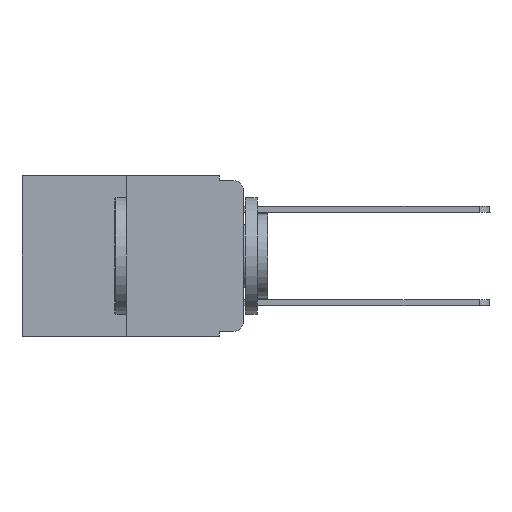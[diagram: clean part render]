
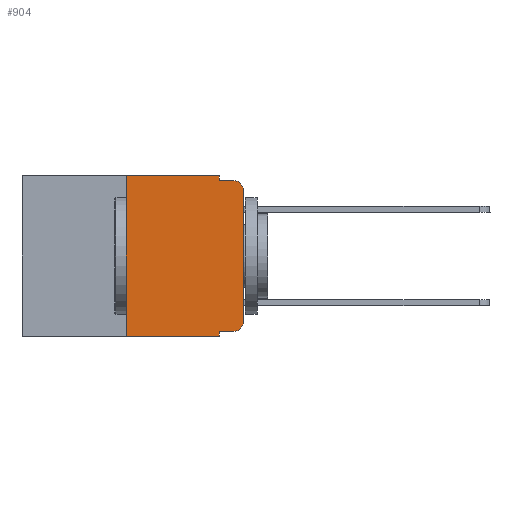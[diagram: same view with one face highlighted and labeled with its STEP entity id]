
A CAD part, left-side view. The second image highlights one B-rep face of the part: STEP entity #904.
In plain terms, the highlighted planar face has unit normal (-1, 0, 0).
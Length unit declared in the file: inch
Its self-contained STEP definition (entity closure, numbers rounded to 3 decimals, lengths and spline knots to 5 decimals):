
#121 = EDGE_CURVE ( 'NONE', #17279, #10276, #17104, .T. ) ;
#374 = CARTESIAN_POINT ( 'NONE',  ( 0., 0.051, -0.333 ) ) ;
#904 = ADVANCED_FACE ( 'NONE', ( #21860 ), #13924, .F. ) ;
#1148 = CARTESIAN_POINT ( 'NONE',  ( 0., 0.473, 0. ) ) ;
#1554 = CIRCLE ( 'NONE', #14560, 0.02 ) ;
#1860 = DIRECTION ( 'NONE',  ( 0., 0., -1. ) ) ;
#1947 = EDGE_CURVE ( 'NONE', #19903, #21428, #14123, .T. ) ;
#2002 = AXIS2_PLACEMENT_3D ( 'NONE', #1148, #24027, #9707 ) ;
#2800 = VECTOR ( 'NONE', #18866, 39.37008 ) ;
#2885 = EDGE_LOOP ( 'NONE', ( #4805, #8491, #22741, #19650, #20838, #8786, #24686, #14273, #6518, #10645 ) ) ;
#3373 = DIRECTION ( 'NONE',  ( -1., 0., 0. ) ) ;
#3546 = VECTOR ( 'NONE', #3890, 39.37008 ) ;
#3624 = CARTESIAN_POINT ( 'NONE',  ( 0., 0., 0. ) ) ;
#3808 = DIRECTION ( 'NONE',  ( 0., -1., 0. ) ) ;
#3831 = CARTESIAN_POINT ( 'NONE',  ( 0., 0.051, 0. ) ) ;
#3858 = VECTOR ( 'NONE', #16967, 39.37008 ) ;
#3890 = DIRECTION ( 'NONE',  ( 0., 0., 1. ) ) ;
#4146 = CARTESIAN_POINT ( 'NONE',  ( 0., 0.051, 0. ) ) ;
#4435 = CARTESIAN_POINT ( 'NONE',  ( 0., 0.25, 0. ) ) ;
#4805 = ORIENTED_EDGE ( 'NONE', *, *, #13808, .T. ) ;
#4909 = EDGE_CURVE ( 'NONE', #5352, #11208, #15163, .T. ) ;
#5352 = VERTEX_POINT ( 'NONE', #6668 ) ;
#5969 = EDGE_CURVE ( 'NONE', #20537, #21428, #16666, .T. ) ;
#6219 = EDGE_CURVE ( 'NONE', #18293, #5352, #23092, .T. ) ;
#6518 = ORIENTED_EDGE ( 'NONE', *, *, #121, .T. ) ;
#6668 = CARTESIAN_POINT ( 'NONE',  ( 0., 0.25, 0. ) ) ;
#7770 = DIRECTION ( 'NONE',  ( 0., 0., -1. ) ) ;
#7827 = LINE ( 'NONE', #3624, #3546 ) ;
#7944 = VECTOR ( 'NONE', #20354, 39.37008 ) ;
#7961 = DIRECTION ( 'NONE',  ( 0., 0., -1. ) ) ;
#8485 = LINE ( 'NONE', #4146, #21129 ) ;
#8491 = ORIENTED_EDGE ( 'NONE', *, *, #5969, .T. ) ;
#8589 = CARTESIAN_POINT ( 'NONE',  ( 0., 0., -0.313 ) ) ;
#8786 = ORIENTED_EDGE ( 'NONE', *, *, #6219, .F. ) ;
#9242 = CARTESIAN_POINT ( 'NONE',  ( 0., 0.051, -0.01 ) ) ;
#9655 = CARTESIAN_POINT ( 'NONE',  ( 0., 0.02, -0.333 ) ) ;
#9665 = LINE ( 'NONE', #3831, #10511 ) ;
#9701 = CARTESIAN_POINT ( 'NONE',  ( 0., 0.473, -0.343 ) ) ;
#9707 = DIRECTION ( 'NONE',  ( 0., 0., -1. ) ) ;
#10141 = VERTEX_POINT ( 'NONE', #8589 ) ;
#10276 = VERTEX_POINT ( 'NONE', #9655 ) ;
#10511 = VECTOR ( 'NONE', #7770, 39.37008 ) ;
#10645 = ORIENTED_EDGE ( 'NONE', *, *, #21133, .T. ) ;
#11208 = VERTEX_POINT ( 'NONE', #21876 ) ;
#11214 = CARTESIAN_POINT ( 'NONE',  ( 0., 0.473, 0. ) ) ;
#13629 = AXIS2_PLACEMENT_3D ( 'NONE', #22030, #3373, #1860 ) ;
#13663 = VECTOR ( 'NONE', #19404, 39.37008 ) ;
#13808 = EDGE_CURVE ( 'NONE', #10141, #20537, #7827, .T. ) ;
#13924 = PLANE ( 'NONE',  #2002 ) ;
#14011 = CARTESIAN_POINT ( 'NONE',  ( 0., 0.02, -0.01 ) ) ;
#14118 = VECTOR ( 'NONE', #3808, 39.37008 ) ;
#14123 = LINE ( 'NONE', #24493, #14118 ) ;
#14273 = ORIENTED_EDGE ( 'NONE', *, *, #16043, .F. ) ;
#14560 = AXIS2_PLACEMENT_3D ( 'NONE', #16646, #26639, #7961 ) ;
#15078 = CARTESIAN_POINT ( 'NONE',  ( 0., 0.051, -0.343 ) ) ;
#15163 = LINE ( 'NONE', #11214, #13663 ) ;
#16043 = EDGE_CURVE ( 'NONE', #17279, #25580, #9665, .T. ) ;
#16390 = DIRECTION ( 'NONE',  ( 0., 0., -1. ) ) ;
#16646 = CARTESIAN_POINT ( 'NONE',  ( 0., 0.02, -0.313 ) ) ;
#16666 = CIRCLE ( 'NONE', #13629, 0.02 ) ;
#16901 = EDGE_CURVE ( 'NONE', #18293, #25580, #26744, .T. ) ;
#16967 = DIRECTION ( 'NONE',  ( 0., -1., 0. ) ) ;
#17104 = LINE ( 'NONE', #374, #3858 ) ;
#17279 = VERTEX_POINT ( 'NONE', #17317 ) ;
#17317 = CARTESIAN_POINT ( 'NONE',  ( 0., 0.051, -0.333 ) ) ;
#18293 = VERTEX_POINT ( 'NONE', #26719 ) ;
#18866 = DIRECTION ( 'NONE',  ( 0., 0., 1. ) ) ;
#19404 = DIRECTION ( 'NONE',  ( 0., -1., 0. ) ) ;
#19650 = ORIENTED_EDGE ( 'NONE', *, *, #21048, .F. ) ;
#19903 = VERTEX_POINT ( 'NONE', #9242 ) ;
#20354 = DIRECTION ( 'NONE',  ( 0., -1., 0. ) ) ;
#20537 = VERTEX_POINT ( 'NONE', #26668 ) ;
#20838 = ORIENTED_EDGE ( 'NONE', *, *, #4909, .F. ) ;
#21048 = EDGE_CURVE ( 'NONE', #11208, #19903, #8485, .T. ) ;
#21129 = VECTOR ( 'NONE', #16390, 39.37008 ) ;
#21133 = EDGE_CURVE ( 'NONE', #10276, #10141, #1554, .T. ) ;
#21428 = VERTEX_POINT ( 'NONE', #14011 ) ;
#21860 = FACE_OUTER_BOUND ( 'NONE', #2885, .T. ) ;
#21876 = CARTESIAN_POINT ( 'NONE',  ( 0., 0.051, 0. ) ) ;
#22030 = CARTESIAN_POINT ( 'NONE',  ( 0., 0.02, -0.03 ) ) ;
#22741 = ORIENTED_EDGE ( 'NONE', *, *, #1947, .F. ) ;
#23092 = LINE ( 'NONE', #4435, #2800 ) ;
#24027 = DIRECTION ( 'NONE',  ( 1., 0., 0. ) ) ;
#24493 = CARTESIAN_POINT ( 'NONE',  ( 0., 0.051, -0.01 ) ) ;
#24686 = ORIENTED_EDGE ( 'NONE', *, *, #16901, .T. ) ;
#25580 = VERTEX_POINT ( 'NONE', #15078 ) ;
#26639 = DIRECTION ( 'NONE',  ( -1., 0., 0. ) ) ;
#26668 = CARTESIAN_POINT ( 'NONE',  ( 0., 0., -0.03 ) ) ;
#26719 = CARTESIAN_POINT ( 'NONE',  ( 0., 0.25, -0.343 ) ) ;
#26744 = LINE ( 'NONE', #9701, #7944 ) ;
